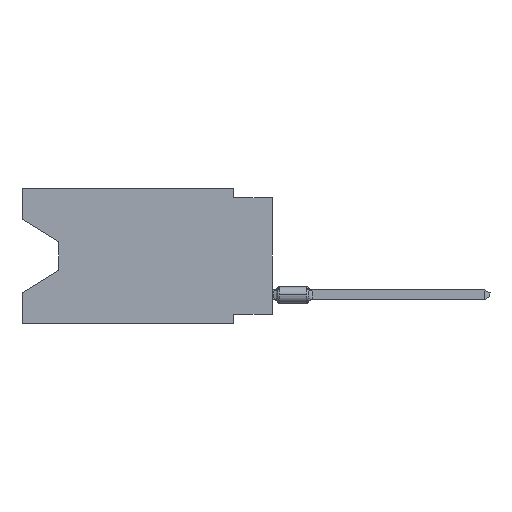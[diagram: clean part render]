
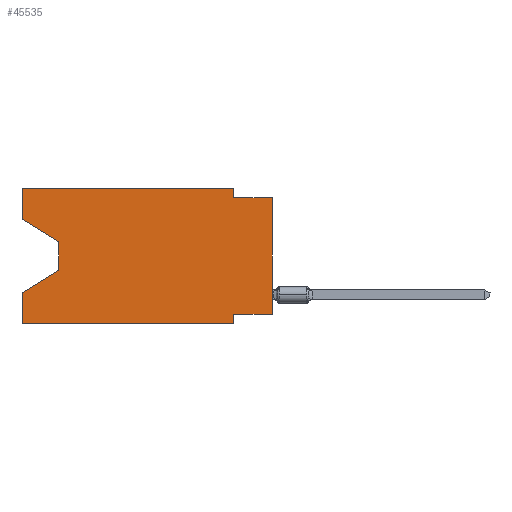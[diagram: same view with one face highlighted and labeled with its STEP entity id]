
A CAD part, left-side view. The second image highlights one B-rep face of the part: STEP entity #45535.
In plain terms, the highlighted planar face has unit normal (-1, 0, 0).
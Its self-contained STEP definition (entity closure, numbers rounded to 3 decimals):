
#415 = LINE ( 'NONE', #32008, #35120 ) ;
#1241 = CARTESIAN_POINT ( 'NONE',  ( 0., 0., -0.635 ) ) ;
#3278 = EDGE_CURVE ( 'NONE', #12482, #44283, #26435, .T. ) ;
#4233 = AXIS2_PLACEMENT_3D ( 'NONE', #57166, #31071, #10153 ) ;
#4478 = DIRECTION ( 'NONE',  ( 0., 0., 1. ) ) ;
#4536 = CARTESIAN_POINT ( 'NONE',  ( 0., 16.383, -2.038 ) ) ;
#5314 = CARTESIAN_POINT ( 'NONE',  ( 0., 16.383, -8.89 ) ) ;
#5627 = VECTOR ( 'NONE', #46422, 1000. ) ;
#5717 = LINE ( 'NONE', #1241, #16081 ) ;
#6742 = DIRECTION ( 'NONE',  ( 0., -1., 0. ) ) ;
#8266 = VERTEX_POINT ( 'NONE', #5314 ) ;
#8789 = EDGE_CURVE ( 'NONE', #8266, #55452, #50158, .T. ) ;
#9455 = FACE_OUTER_BOUND ( 'NONE', #33417, .T. ) ;
#10153 = DIRECTION ( 'NONE',  ( 0., 0., -1. ) ) ;
#10180 = EDGE_CURVE ( 'NONE', #56639, #55452, #33129, .T. ) ;
#11809 = ORIENTED_EDGE ( 'NONE', *, *, #26335, .T. ) ;
#12482 = VERTEX_POINT ( 'NONE', #28036 ) ;
#12516 = CARTESIAN_POINT ( 'NONE',  ( 0., 13.97, -3.505 ) ) ;
#13773 = CARTESIAN_POINT ( 'NONE',  ( 0., 2.54, -8.255 ) ) ;
#14118 = VECTOR ( 'NONE', #36295, 1000. ) ;
#14982 = ORIENTED_EDGE ( 'NONE', *, *, #24409, .F. ) ;
#15348 = DIRECTION ( 'NONE',  ( 0., 0., 1. ) ) ;
#15501 = ORIENTED_EDGE ( 'NONE', *, *, #64509, .T. ) ;
#16067 = CARTESIAN_POINT ( 'NONE',  ( 0., 16.383, -2.038 ) ) ;
#16081 = VECTOR ( 'NONE', #6742, 1000. ) ;
#16189 = ORIENTED_EDGE ( 'NONE', *, *, #10180, .T. ) ;
#18364 = VERTEX_POINT ( 'NONE', #13773 ) ;
#20242 = LINE ( 'NONE', #36009, #56437 ) ;
#22580 = CARTESIAN_POINT ( 'NONE',  ( 0., 16.383, 0. ) ) ;
#22762 = CARTESIAN_POINT ( 'NONE',  ( 0., 13.97, -5.385 ) ) ;
#23730 = DIRECTION ( 'NONE',  ( 0., 0., 1. ) ) ;
#24409 = EDGE_CURVE ( 'NONE', #18364, #36643, #20242, .T. ) ;
#25447 = EDGE_CURVE ( 'NONE', #12482, #18364, #29360, .T. ) ;
#26036 = VERTEX_POINT ( 'NONE', #54035 ) ;
#26076 = CARTESIAN_POINT ( 'NONE',  ( 0., 0., 0. ) ) ;
#26335 = EDGE_CURVE ( 'NONE', #39178, #66400, #63544, .T. ) ;
#26435 = LINE ( 'NONE', #26076, #29789 ) ;
#27133 = CARTESIAN_POINT ( 'NONE',  ( 0., 2.54, -8.89 ) ) ;
#27255 = VECTOR ( 'NONE', #49731, 1000. ) ;
#28036 = CARTESIAN_POINT ( 'NONE',  ( 0., 0., -8.255 ) ) ;
#28781 = LINE ( 'NONE', #50746, #27255 ) ;
#29010 = EDGE_CURVE ( 'NONE', #39178, #43917, #29118, .T. ) ;
#29118 = LINE ( 'NONE', #44903, #56719 ) ;
#29360 = LINE ( 'NONE', #54776, #52677 ) ;
#29789 = VECTOR ( 'NONE', #4478, 1000. ) ;
#31071 = DIRECTION ( 'NONE',  ( 1., 0., 0. ) ) ;
#31718 = VECTOR ( 'NONE', #23730, 1000. ) ;
#32008 = CARTESIAN_POINT ( 'NONE',  ( 0., 16.383, 0. ) ) ;
#33055 = ORIENTED_EDGE ( 'NONE', *, *, #25447, .F. ) ;
#33129 = LINE ( 'NONE', #47889, #45018 ) ;
#33417 = EDGE_LOOP ( 'NONE', ( #11809, #49109, #16189, #48430, #15501, #14982, #33055, #59052, #51191, #55140, #57470, #57761 ) ) ;
#34036 = CARTESIAN_POINT ( 'NONE',  ( 0., 16.383, 0. ) ) ;
#34840 = DIRECTION ( 'NONE',  ( 0., 1., 0. ) ) ;
#35120 = VECTOR ( 'NONE', #63918, 1000. ) ;
#36009 = CARTESIAN_POINT ( 'NONE',  ( 0., 2.54, -8.89 ) ) ;
#36295 = DIRECTION ( 'NONE',  ( 0., 0., -1. ) ) ;
#36643 = VERTEX_POINT ( 'NONE', #27133 ) ;
#39178 = VERTEX_POINT ( 'NONE', #16067 ) ;
#43917 = VERTEX_POINT ( 'NONE', #22580 ) ;
#44283 = VERTEX_POINT ( 'NONE', #53736 ) ;
#44692 = DIRECTION ( 'NONE',  ( 0., 0., -1. ) ) ;
#44903 = CARTESIAN_POINT ( 'NONE',  ( 0., 16.383, 0. ) ) ;
#45018 = VECTOR ( 'NONE', #48920, 1000. ) ;
#45387 = CARTESIAN_POINT ( 'NONE',  ( 0., 16.383, -6.852 ) ) ;
#45535 = ADVANCED_FACE ( 'NONE', ( #9455 ), #56805, .F. ) ;
#46422 = DIRECTION ( 'NONE',  ( 0., -0.855, -0.519 ) ) ;
#47742 = VECTOR ( 'NONE', #44692, 1000. ) ;
#47889 = CARTESIAN_POINT ( 'NONE',  ( 0., 13.97, -5.385 ) ) ;
#48430 = ORIENTED_EDGE ( 'NONE', *, *, #8789, .F. ) ;
#48829 = EDGE_CURVE ( 'NONE', #43917, #26036, #415, .T. ) ;
#48920 = DIRECTION ( 'NONE',  ( 0., 0.855, -0.519 ) ) ;
#49109 = ORIENTED_EDGE ( 'NONE', *, *, #64630, .T. ) ;
#49191 = CARTESIAN_POINT ( 'NONE',  ( 0., 2.54, -0.635 ) ) ;
#49731 = DIRECTION ( 'NONE',  ( 0., -1., 0. ) ) ;
#49858 = CARTESIAN_POINT ( 'NONE',  ( 0., 2.54, 0. ) ) ;
#50158 = LINE ( 'NONE', #34036, #31718 ) ;
#50746 = CARTESIAN_POINT ( 'NONE',  ( 0., 16.383, -8.89 ) ) ;
#51191 = ORIENTED_EDGE ( 'NONE', *, *, #62353, .F. ) ;
#51901 = VERTEX_POINT ( 'NONE', #49191 ) ;
#52677 = VECTOR ( 'NONE', #34840, 1000. ) ;
#52954 = EDGE_CURVE ( 'NONE', #26036, #51901, #56022, .T. ) ;
#53736 = CARTESIAN_POINT ( 'NONE',  ( 0., 0., -0.635 ) ) ;
#54035 = CARTESIAN_POINT ( 'NONE',  ( 0., 2.54, 0. ) ) ;
#54776 = CARTESIAN_POINT ( 'NONE',  ( 0., 0., -8.255 ) ) ;
#55140 = ORIENTED_EDGE ( 'NONE', *, *, #52954, .F. ) ;
#55452 = VERTEX_POINT ( 'NONE', #45387 ) ;
#56022 = LINE ( 'NONE', #49858, #47742 ) ;
#56437 = VECTOR ( 'NONE', #56963, 1000. ) ;
#56639 = VERTEX_POINT ( 'NONE', #22762 ) ;
#56719 = VECTOR ( 'NONE', #15348, 1000. ) ;
#56805 = PLANE ( 'NONE',  #4233 ) ;
#56963 = DIRECTION ( 'NONE',  ( 0., 0., -1. ) ) ;
#57166 = CARTESIAN_POINT ( 'NONE',  ( 0., 16.383, 0. ) ) ;
#57470 = ORIENTED_EDGE ( 'NONE', *, *, #48829, .F. ) ;
#57761 = ORIENTED_EDGE ( 'NONE', *, *, #29010, .F. ) ;
#59052 = ORIENTED_EDGE ( 'NONE', *, *, #3278, .T. ) ;
#61698 = LINE ( 'NONE', #62024, #14118 ) ;
#62024 = CARTESIAN_POINT ( 'NONE',  ( 0., 13.97, -3.505 ) ) ;
#62353 = EDGE_CURVE ( 'NONE', #51901, #44283, #5717, .T. ) ;
#63544 = LINE ( 'NONE', #4536, #5627 ) ;
#63918 = DIRECTION ( 'NONE',  ( 0., -1., 0. ) ) ;
#64509 = EDGE_CURVE ( 'NONE', #8266, #36643, #28781, .T. ) ;
#64630 = EDGE_CURVE ( 'NONE', #66400, #56639, #61698, .T. ) ;
#66400 = VERTEX_POINT ( 'NONE', #12516 ) ;
